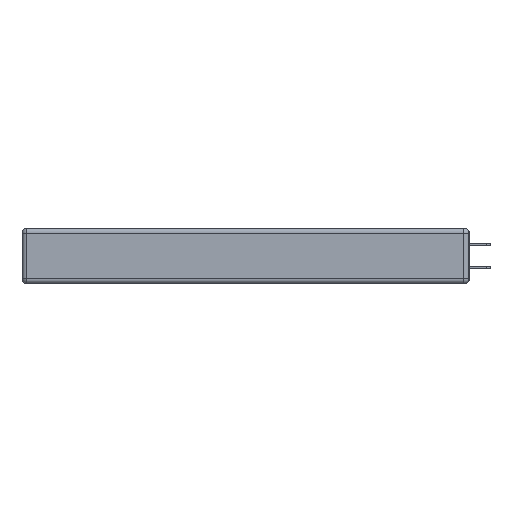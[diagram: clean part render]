
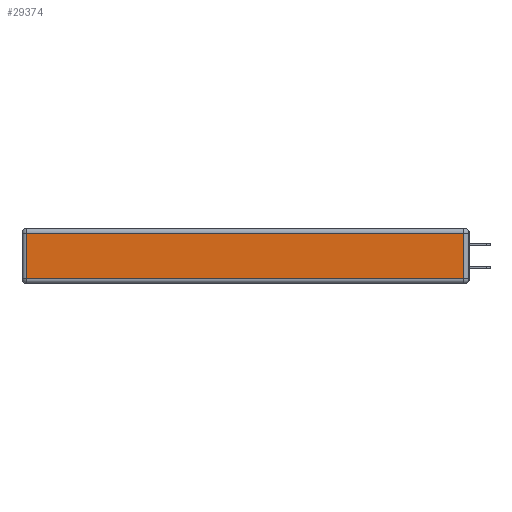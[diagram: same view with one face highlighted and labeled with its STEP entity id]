
A CAD part, left-side view. The second image highlights one B-rep face of the part: STEP entity #29374.
In plain terms, the highlighted planar face has unit normal (-1, 0, 0).
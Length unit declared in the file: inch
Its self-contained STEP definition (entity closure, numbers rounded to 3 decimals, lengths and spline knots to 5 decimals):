
#1075 = CARTESIAN_POINT ( 'NONE',  ( 0., 2.72, -0.03 ) ) ;
#3305 = ORIENTED_EDGE ( 'NONE', *, *, #22209, .T. ) ;
#3545 = EDGE_CURVE ( 'NONE', #12580, #8460, #25828, .T. ) ;
#4326 = LINE ( 'NONE', #21319, #11762 ) ;
#5104 = CARTESIAN_POINT ( 'NONE',  ( 0., 0.03, -0.03 ) ) ;
#6333 = VERTEX_POINT ( 'NONE', #1075 ) ;
#6604 = FACE_OUTER_BOUND ( 'NONE', #21384, .T. ) ;
#7768 = PLANE ( 'NONE',  #12334 ) ;
#8460 = VERTEX_POINT ( 'NONE', #29390 ) ;
#9832 = CARTESIAN_POINT ( 'NONE',  ( 0., 0., -0.343 ) ) ;
#10169 = ORIENTED_EDGE ( 'NONE', *, *, #28373, .T. ) ;
#11762 = VECTOR ( 'NONE', #16862, 39.37008 ) ;
#12334 = AXIS2_PLACEMENT_3D ( 'NONE', #9832, #24035, #24133 ) ;
#12580 = VERTEX_POINT ( 'NONE', #28057 ) ;
#15217 = CARTESIAN_POINT ( 'NONE',  ( 0., 0., -0.313 ) ) ;
#16658 = ORIENTED_EDGE ( 'NONE', *, *, #30430, .T. ) ;
#16862 = DIRECTION ( 'NONE',  ( 0., 0., 1. ) ) ;
#16906 = DIRECTION ( 'NONE',  ( 0., 0., -1. ) ) ;
#17633 = DIRECTION ( 'NONE',  ( 0., -1., 0. ) ) ;
#17997 = CARTESIAN_POINT ( 'NONE',  ( 0., 2.75, -0.03 ) ) ;
#19386 = CARTESIAN_POINT ( 'NONE',  ( 0., 2.72, -0.343 ) ) ;
#20624 = ORIENTED_EDGE ( 'NONE', *, *, #3545, .T. ) ;
#20953 = VERTEX_POINT ( 'NONE', #5104 ) ;
#21319 = CARTESIAN_POINT ( 'NONE',  ( 0., 0.03, -0.343 ) ) ;
#21384 = EDGE_LOOP ( 'NONE', ( #20624, #16658, #10169, #3305 ) ) ;
#22209 = EDGE_CURVE ( 'NONE', #6333, #12580, #22983, .T. ) ;
#22983 = LINE ( 'NONE', #19386, #28553 ) ;
#24035 = DIRECTION ( 'NONE',  ( -1., 0., 0. ) ) ;
#24054 = VECTOR ( 'NONE', #29760, 39.37008 ) ;
#24133 = DIRECTION ( 'NONE',  ( 0., 0., 1. ) ) ;
#25828 = LINE ( 'NONE', #15217, #28787 ) ;
#28057 = CARTESIAN_POINT ( 'NONE',  ( 0., 2.72, -0.313 ) ) ;
#28373 = EDGE_CURVE ( 'NONE', #20953, #6333, #29213, .T. ) ;
#28553 = VECTOR ( 'NONE', #16906, 39.37008 ) ;
#28787 = VECTOR ( 'NONE', #17633, 39.37008 ) ;
#29213 = LINE ( 'NONE', #17997, #24054 ) ;
#29374 = ADVANCED_FACE ( 'NONE', ( #6604 ), #7768, .T. ) ;
#29390 = CARTESIAN_POINT ( 'NONE',  ( 0., 0.03, -0.313 ) ) ;
#29760 = DIRECTION ( 'NONE',  ( 0., 1., 0. ) ) ;
#30430 = EDGE_CURVE ( 'NONE', #8460, #20953, #4326, .T. ) ;
